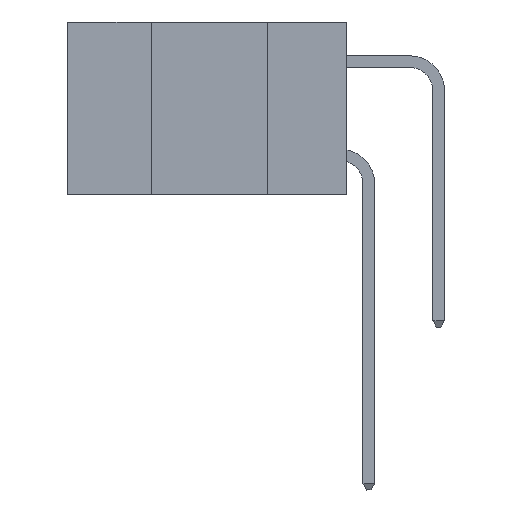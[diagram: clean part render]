
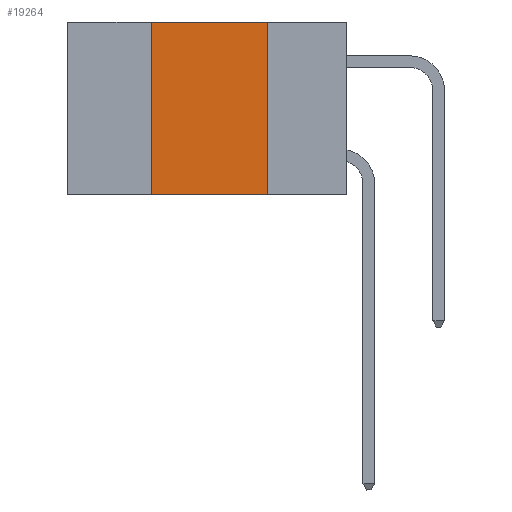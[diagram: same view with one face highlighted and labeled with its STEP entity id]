
A CAD part, left-side view. The second image highlights one B-rep face of the part: STEP entity #19264.
In plain terms, the highlighted planar face has unit normal (-1, 0, 0).
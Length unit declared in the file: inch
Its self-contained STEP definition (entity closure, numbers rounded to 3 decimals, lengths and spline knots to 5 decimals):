
#63 = EDGE_CURVE ( 'NONE', #13573, #4767, #25184, .T. ) ;
#574 = VERTEX_POINT ( 'NONE', #7106 ) ;
#586 = CARTESIAN_POINT ( 'NONE',  ( 0., 0.42, 0. ) ) ;
#897 = CARTESIAN_POINT ( 'NONE',  ( 0., 0.6, 0. ) ) ;
#1291 = EDGE_CURVE ( 'NONE', #13573, #14587, #24149, .T. ) ;
#4767 = VERTEX_POINT ( 'NONE', #586 ) ;
#5369 = DIRECTION ( 'NONE',  ( 0., 0., -1. ) ) ;
#7106 = CARTESIAN_POINT ( 'NONE',  ( 0., 0.17, 0. ) ) ;
#8963 = CARTESIAN_POINT ( 'NONE',  ( 0., 0.6, 0. ) ) ;
#10163 = FACE_OUTER_BOUND ( 'NONE', #16263, .T. ) ;
#11059 = DIRECTION ( 'NONE',  ( 0., 0., -1. ) ) ;
#11728 = LINE ( 'NONE', #26460, #22381 ) ;
#13573 = VERTEX_POINT ( 'NONE', #24753 ) ;
#14587 = VERTEX_POINT ( 'NONE', #23050 ) ;
#16263 = EDGE_LOOP ( 'NONE', ( #25571, #20701, #26852, #16349 ) ) ;
#16349 = ORIENTED_EDGE ( 'NONE', *, *, #1291, .T. ) ;
#18044 = DIRECTION ( 'NONE',  ( 0., -1., 0. ) ) ;
#18358 = DIRECTION ( 'NONE',  ( 0., 0., 1. ) ) ;
#18601 = VECTOR ( 'NONE', #25937, 39.37008 ) ;
#19009 = VECTOR ( 'NONE', #18358, 39.37008 ) ;
#19264 = ADVANCED_FACE ( 'NONE', ( #10163 ), #21678, .F. ) ;
#19695 = LINE ( 'NONE', #897, #25211 ) ;
#20701 = ORIENTED_EDGE ( 'NONE', *, *, #21561, .F. ) ;
#21561 = EDGE_CURVE ( 'NONE', #4767, #574, #19695, .T. ) ;
#21678 = PLANE ( 'NONE',  #25940 ) ;
#22381 = VECTOR ( 'NONE', #5369, 39.37008 ) ;
#23050 = CARTESIAN_POINT ( 'NONE',  ( 0., 0.17, -0.37 ) ) ;
#23758 = DIRECTION ( 'NONE',  ( 1., 0., 0. ) ) ;
#24149 = LINE ( 'NONE', #25477, #18601 ) ;
#24553 = CARTESIAN_POINT ( 'NONE',  ( 0., 0.42, 0. ) ) ;
#24753 = CARTESIAN_POINT ( 'NONE',  ( 0., 0.42, -0.37 ) ) ;
#25184 = LINE ( 'NONE', #24553, #19009 ) ;
#25211 = VECTOR ( 'NONE', #18044, 39.37008 ) ;
#25477 = CARTESIAN_POINT ( 'NONE',  ( 0., 0.6, -0.37 ) ) ;
#25571 = ORIENTED_EDGE ( 'NONE', *, *, #26349, .F. ) ;
#25937 = DIRECTION ( 'NONE',  ( 0., -1., 0. ) ) ;
#25940 = AXIS2_PLACEMENT_3D ( 'NONE', #8963, #23758, #11059 ) ;
#26349 = EDGE_CURVE ( 'NONE', #574, #14587, #11728, .T. ) ;
#26460 = CARTESIAN_POINT ( 'NONE',  ( 0., 0.17, 0. ) ) ;
#26852 = ORIENTED_EDGE ( 'NONE', *, *, #63, .F. ) ;
